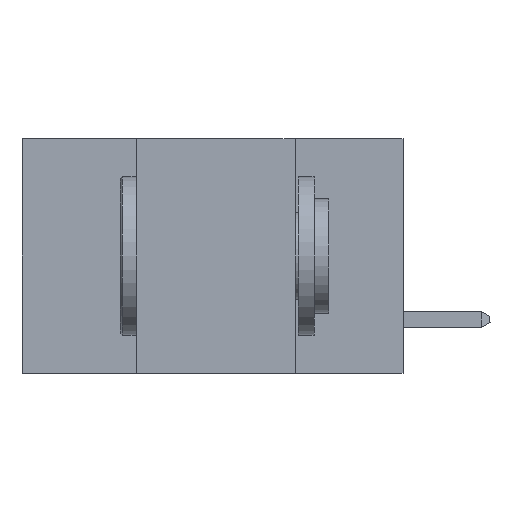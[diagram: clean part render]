
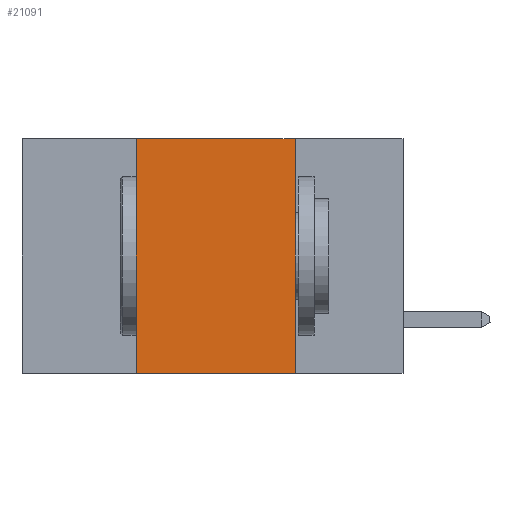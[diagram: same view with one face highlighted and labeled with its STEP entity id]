
A CAD part, left-side view. The second image highlights one B-rep face of the part: STEP entity #21091.
In plain terms, the highlighted planar face has unit normal (-1, 0, 0).
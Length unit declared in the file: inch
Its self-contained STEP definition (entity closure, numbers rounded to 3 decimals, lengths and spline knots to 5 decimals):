
#550 = CARTESIAN_POINT ( 'NONE',  ( 0., 0.6, 0. ) ) ;
#1441 = VECTOR ( 'NONE', #2558, 39.37008 ) ;
#2289 = ORIENTED_EDGE ( 'NONE', *, *, #22844, .F. ) ;
#2558 = DIRECTION ( 'NONE',  ( 0., -1., 0. ) ) ;
#4138 = EDGE_CURVE ( 'NONE', #20410, #16657, #14614, .T. ) ;
#4588 = ORIENTED_EDGE ( 'NONE', *, *, #4138, .T. ) ;
#4794 = FACE_OUTER_BOUND ( 'NONE', #24772, .T. ) ;
#6165 = DIRECTION ( 'NONE',  ( 0., -1., 0. ) ) ;
#6195 = LINE ( 'NONE', #12721, #21699 ) ;
#6267 = DIRECTION ( 'NONE',  ( 1., 0., 0. ) ) ;
#7619 = CARTESIAN_POINT ( 'NONE',  ( 0., 0.17, 0. ) ) ;
#8713 = VECTOR ( 'NONE', #6165, 39.37008 ) ;
#9789 = CARTESIAN_POINT ( 'NONE',  ( 0., 0.6, -0.37 ) ) ;
#10356 = ORIENTED_EDGE ( 'NONE', *, *, #11325, .F. ) ;
#10396 = PLANE ( 'NONE',  #17462 ) ;
#11325 = EDGE_CURVE ( 'NONE', #22429, #19442, #23146, .T. ) ;
#12115 = CARTESIAN_POINT ( 'NONE',  ( 0., 0.17, 0. ) ) ;
#12564 = CARTESIAN_POINT ( 'NONE',  ( 0., 0.6, 0. ) ) ;
#12721 = CARTESIAN_POINT ( 'NONE',  ( 0., 0.42, 0. ) ) ;
#14614 = LINE ( 'NONE', #9789, #8713 ) ;
#16657 = VERTEX_POINT ( 'NONE', #21909 ) ;
#16712 = DIRECTION ( 'NONE',  ( 0., 0., 1. ) ) ;
#17462 = AXIS2_PLACEMENT_3D ( 'NONE', #12564, #6267, #20132 ) ;
#18463 = LINE ( 'NONE', #7619, #18783 ) ;
#18783 = VECTOR ( 'NONE', #21780, 39.37008 ) ;
#19442 = VERTEX_POINT ( 'NONE', #12115 ) ;
#20132 = DIRECTION ( 'NONE',  ( 0., 0., -1. ) ) ;
#20410 = VERTEX_POINT ( 'NONE', #23106 ) ;
#21091 = ADVANCED_FACE ( 'NONE', ( #4794 ), #10396, .F. ) ;
#21699 = VECTOR ( 'NONE', #16712, 39.37008 ) ;
#21780 = DIRECTION ( 'NONE',  ( 0., 0., -1. ) ) ;
#21909 = CARTESIAN_POINT ( 'NONE',  ( 0., 0.17, -0.37 ) ) ;
#22136 = ORIENTED_EDGE ( 'NONE', *, *, #25504, .F. ) ;
#22429 = VERTEX_POINT ( 'NONE', #25034 ) ;
#22844 = EDGE_CURVE ( 'NONE', #20410, #22429, #6195, .T. ) ;
#23106 = CARTESIAN_POINT ( 'NONE',  ( 0., 0.42, -0.37 ) ) ;
#23146 = LINE ( 'NONE', #550, #1441 ) ;
#24772 = EDGE_LOOP ( 'NONE', ( #22136, #10356, #2289, #4588 ) ) ;
#25034 = CARTESIAN_POINT ( 'NONE',  ( 0., 0.42, 0. ) ) ;
#25504 = EDGE_CURVE ( 'NONE', #19442, #16657, #18463, .T. ) ;
